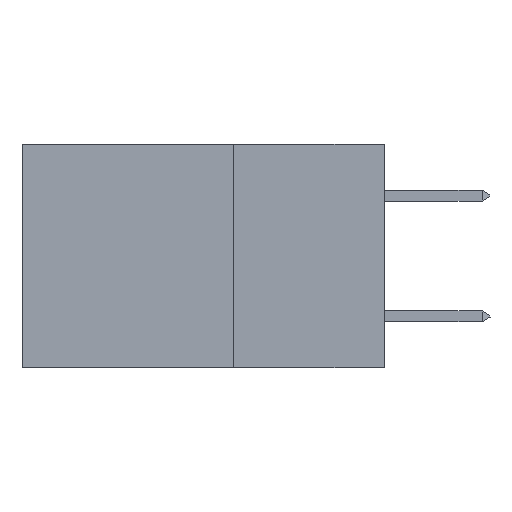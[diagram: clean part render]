
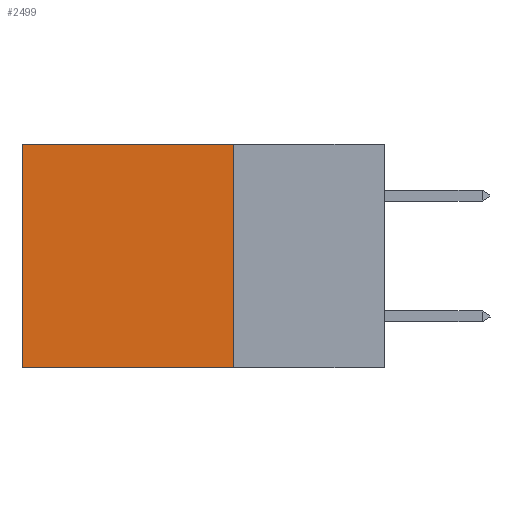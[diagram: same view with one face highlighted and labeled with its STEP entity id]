
A CAD part, left-side view. The second image highlights one B-rep face of the part: STEP entity #2499.
In plain terms, the highlighted planar face has unit normal (-1, 0, 0).
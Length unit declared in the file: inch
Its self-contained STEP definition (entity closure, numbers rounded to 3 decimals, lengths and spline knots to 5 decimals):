
#23 = CARTESIAN_POINT ( 'NONE',  ( 0.2875, 0.25, 0. ) ) ;
#152 = LINE ( 'NONE', #23, #2860 ) ;
#507 = CARTESIAN_POINT ( 'NONE',  ( 0.2875, 0.6, -0.37 ) ) ;
#515 = CARTESIAN_POINT ( 'NONE',  ( 0.2875, 0.6, 0. ) ) ;
#813 = EDGE_LOOP ( 'NONE', ( #9832, #8628, #3620, #14853 ) ) ;
#905 = FACE_OUTER_BOUND ( 'NONE', #813, .T. ) ;
#2040 = CARTESIAN_POINT ( 'NONE',  ( 0.2875, 0.6, 0. ) ) ;
#2499 = ADVANCED_FACE ( 'NONE', ( #905 ), #3904, .F. ) ;
#2860 = VECTOR ( 'NONE', #9039, 39.37008 ) ;
#3269 = LINE ( 'NONE', #3821, #3615 ) ;
#3615 = VECTOR ( 'NONE', #14045, 39.37008 ) ;
#3620 = ORIENTED_EDGE ( 'NONE', *, *, #7924, .F. ) ;
#3821 = CARTESIAN_POINT ( 'NONE',  ( 0.2875, 0.25, -0.37 ) ) ;
#3904 = PLANE ( 'NONE',  #14798 ) ;
#3938 = VERTEX_POINT ( 'NONE', #2040 ) ;
#3960 = DIRECTION ( 'NONE',  ( 1., 0., 0. ) ) ;
#4051 = VECTOR ( 'NONE', #14384, 39.37008 ) ;
#5196 = CARTESIAN_POINT ( 'NONE',  ( 0.2875, 0.25, 0. ) ) ;
#5296 = EDGE_CURVE ( 'NONE', #6680, #3938, #152, .T. ) ;
#6131 = CARTESIAN_POINT ( 'NONE',  ( 0.2875, 0.25, 0. ) ) ;
#6680 = VERTEX_POINT ( 'NONE', #13670 ) ;
#7016 = EDGE_CURVE ( 'NONE', #3938, #11678, #11632, .T. ) ;
#7924 = EDGE_CURVE ( 'NONE', #6680, #10880, #13228, .T. ) ;
#8628 = ORIENTED_EDGE ( 'NONE', *, *, #9715, .F. ) ;
#9039 = DIRECTION ( 'NONE',  ( 0., 1., 0. ) ) ;
#9702 = DIRECTION ( 'NONE',  ( 0., 0., -1. ) ) ;
#9715 = EDGE_CURVE ( 'NONE', #10880, #11678, #3269, .T. ) ;
#9832 = ORIENTED_EDGE ( 'NONE', *, *, #7016, .T. ) ;
#10841 = DIRECTION ( 'NONE',  ( 0., 0., -1. ) ) ;
#10880 = VERTEX_POINT ( 'NONE', #12966 ) ;
#11632 = LINE ( 'NONE', #515, #12863 ) ;
#11678 = VERTEX_POINT ( 'NONE', #507 ) ;
#12863 = VECTOR ( 'NONE', #10841, 39.37008 ) ;
#12966 = CARTESIAN_POINT ( 'NONE',  ( 0.2875, 0.25, -0.37 ) ) ;
#13228 = LINE ( 'NONE', #5196, #4051 ) ;
#13670 = CARTESIAN_POINT ( 'NONE',  ( 0.2875, 0.25, 0. ) ) ;
#14045 = DIRECTION ( 'NONE',  ( 0., 1., 0. ) ) ;
#14384 = DIRECTION ( 'NONE',  ( 0., 0., -1. ) ) ;
#14798 = AXIS2_PLACEMENT_3D ( 'NONE', #6131, #3960, #9702 ) ;
#14853 = ORIENTED_EDGE ( 'NONE', *, *, #5296, .T. ) ;
